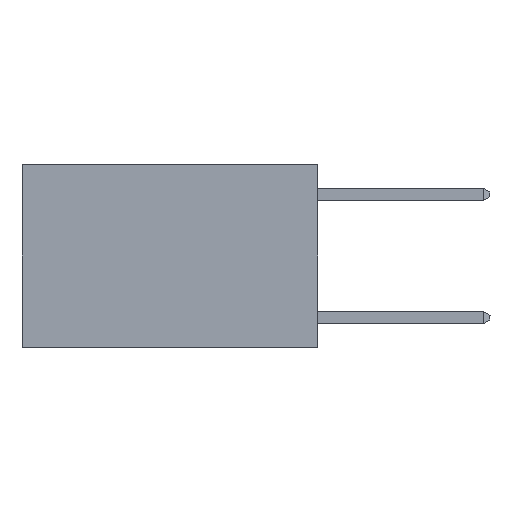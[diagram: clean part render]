
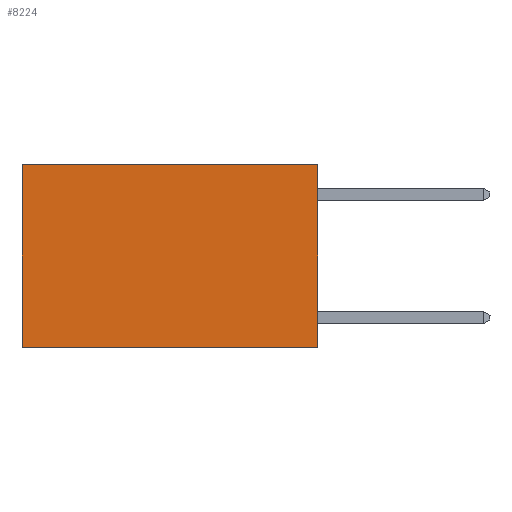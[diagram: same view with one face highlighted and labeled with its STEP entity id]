
A CAD part, left-side view. The second image highlights one B-rep face of the part: STEP entity #8224.
In plain terms, the highlighted planar face has unit normal (-1, 0, 0).
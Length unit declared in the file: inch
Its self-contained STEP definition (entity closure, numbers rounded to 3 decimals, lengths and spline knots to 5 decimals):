
#2730 = CARTESIAN_POINT ( 'NONE',  ( 0.2625, 0., -0.37 ) ) ;
#2731 = DIRECTION ( 'NONE',  ( 0., 1., 0. ) ) ;
#3074 = VECTOR ( 'NONE', #25878, 39.37008 ) ;
#3737 = VERTEX_POINT ( 'NONE', #23185 ) ;
#3879 = EDGE_LOOP ( 'NONE', ( #25659, #10567, #16716, #14614 ) ) ;
#4979 = EDGE_CURVE ( 'NONE', #10566, #3737, #7413, .T. ) ;
#7413 = LINE ( 'NONE', #11442, #17061 ) ;
#7512 = LINE ( 'NONE', #13341, #9772 ) ;
#7948 = CARTESIAN_POINT ( 'NONE',  ( 0.2625, 0., 0. ) ) ;
#8224 = ADVANCED_FACE ( 'NONE', ( #13259 ), #9304, .F. ) ;
#9216 = DIRECTION ( 'NONE',  ( 1., 0., 0. ) ) ;
#9304 = PLANE ( 'NONE',  #23789 ) ;
#9772 = VECTOR ( 'NONE', #2731, 39.37008 ) ;
#10030 = VERTEX_POINT ( 'NONE', #2730 ) ;
#10566 = VERTEX_POINT ( 'NONE', #7948 ) ;
#10567 = ORIENTED_EDGE ( 'NONE', *, *, #26360, .F. ) ;
#10636 = LINE ( 'NONE', #21716, #20916 ) ;
#11442 = CARTESIAN_POINT ( 'NONE',  ( 0.2625, 0., 0. ) ) ;
#11841 = DIRECTION ( 'NONE',  ( 0., 0., -1. ) ) ;
#13259 = FACE_OUTER_BOUND ( 'NONE', #3879, .T. ) ;
#13341 = CARTESIAN_POINT ( 'NONE',  ( 0.2625, 0., -0.37 ) ) ;
#14614 = ORIENTED_EDGE ( 'NONE', *, *, #4979, .T. ) ;
#15225 = CARTESIAN_POINT ( 'NONE',  ( 0.2625, 0., 0. ) ) ;
#16716 = ORIENTED_EDGE ( 'NONE', *, *, #25206, .F. ) ;
#16904 = CARTESIAN_POINT ( 'NONE',  ( 0.2625, 0.6, -0.37 ) ) ;
#17061 = VECTOR ( 'NONE', #25819, 39.37008 ) ;
#17538 = LINE ( 'NONE', #17697, #3074 ) ;
#17697 = CARTESIAN_POINT ( 'NONE',  ( 0.2625, 0., 0. ) ) ;
#17913 = EDGE_CURVE ( 'NONE', #3737, #22670, #10636, .T. ) ;
#20916 = VECTOR ( 'NONE', #11841, 39.37008 ) ;
#21716 = CARTESIAN_POINT ( 'NONE',  ( 0.2625, 0.6, 0. ) ) ;
#22670 = VERTEX_POINT ( 'NONE', #16904 ) ;
#23185 = CARTESIAN_POINT ( 'NONE',  ( 0.2625, 0.6, 0. ) ) ;
#23416 = DIRECTION ( 'NONE',  ( 0., 0., -1. ) ) ;
#23789 = AXIS2_PLACEMENT_3D ( 'NONE', #15225, #9216, #23416 ) ;
#25206 = EDGE_CURVE ( 'NONE', #10566, #10030, #17538, .T. ) ;
#25659 = ORIENTED_EDGE ( 'NONE', *, *, #17913, .T. ) ;
#25819 = DIRECTION ( 'NONE',  ( 0., 1., 0. ) ) ;
#25878 = DIRECTION ( 'NONE',  ( 0., 0., -1. ) ) ;
#26360 = EDGE_CURVE ( 'NONE', #10030, #22670, #7512, .T. ) ;
